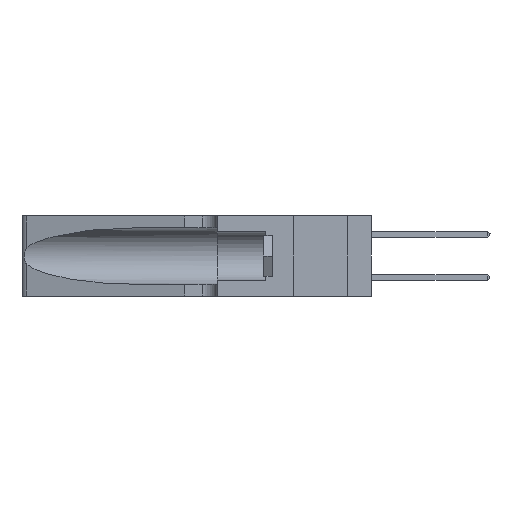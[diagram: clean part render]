
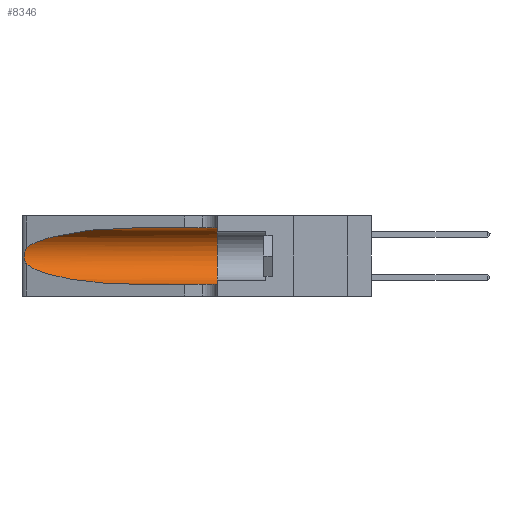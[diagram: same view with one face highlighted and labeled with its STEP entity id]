
A CAD part, left-side view. The second image highlights one B-rep face of the part: STEP entity #8346.
In plain terms, the highlighted cylindrical face has radius 3.308 mm (diameter 6.617 mm), a partial arc.
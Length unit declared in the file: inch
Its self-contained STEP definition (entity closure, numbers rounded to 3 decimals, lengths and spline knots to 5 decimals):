
#1236 = CARTESIAN_POINT ( 'NONE',  ( 0.25639, 1.23184, 0.21858 ) ) ;
#1333 =( BOUNDED_CURVE ( )  B_SPLINE_CURVE ( 3, ( #10373, #8876, #10526, #2086 ),
 .UNSPECIFIED., .F., .T. ) 
 B_SPLINE_CURVE_WITH_KNOTS ( ( 4, 4 ),
 ( 3.44316, 4.71239 ),
 .UNSPECIFIED. ) 
 CURVE ( )  GEOMETRIC_REPRESENTATION_ITEM ( )  RATIONAL_B_SPLINE_CURVE ( ( 1., 0.87, 0.87, 1. ) ) 
 REPRESENTATION_ITEM ( '' )  );
#1506 = CARTESIAN_POINT ( 'NONE',  ( 0.1305, 0.35, 0.185 ) ) ;
#1626 = AXIS2_PLACEMENT_3D ( 'NONE', #2397, #3921, #17804 ) ;
#1773 = CARTESIAN_POINT ( 'NONE',  ( 0.1305, 0.72297, 0.31525 ) ) ;
#2086 = CARTESIAN_POINT ( 'NONE',  ( 0.1305, 0.72297, 0.05475 ) ) ;
#2121 = ORIENTED_EDGE ( 'NONE', *, *, #9922, .T. ) ;
#2397 = CARTESIAN_POINT ( 'NONE',  ( 0.1305, 1.61858, 0.185 ) ) ;
#2415 = VERTEX_POINT ( 'NONE', #15069 ) ;
#2681 = CARTESIAN_POINT ( 'NONE',  ( 0.1305, 0.72297, 0.31525 ) ) ;
#2907 = CARTESIAN_POINT ( 'NONE',  ( 0.1305, 0.35, 0.31525 ) ) ;
#3198 = CARTESIAN_POINT ( 'NONE',  ( 0.26075, 1.23896, 0.19203 ) ) ;
#3245 = DIRECTION ( 'NONE',  ( 0., 0., 1. ) ) ;
#3446 = CARTESIAN_POINT ( 'NONE',  ( 0.2373, 1.15595, 0.28018 ) ) ;
#3921 = DIRECTION ( 'NONE',  ( 0., -1., 0. ) ) ;
#3967 =( BOUNDED_CURVE ( )  B_SPLINE_CURVE ( 3, ( #1773, #13787, #3446, #15420 ),
 .UNSPECIFIED., .F., .T. ) 
 B_SPLINE_CURVE_WITH_KNOTS ( ( 4, 4 ),
 ( 1.5708, 2.84003 ),
 .UNSPECIFIED. ) 
 CURVE ( )  GEOMETRIC_REPRESENTATION_ITEM ( )  RATIONAL_B_SPLINE_CURVE ( ( 1., 0.87, 0.87, 1. ) ) 
 REPRESENTATION_ITEM ( '' )  );
#4155 = EDGE_CURVE ( 'NONE', #12718, #6421, #21612, .T. ) ;
#4367 = ORIENTED_EDGE ( 'NONE', *, *, #4155, .T. ) ;
#4467 = CARTESIAN_POINT ( 'NONE',  ( 0.25487, 1.22718, 0.22369 ) ) ;
#4533 = CARTESIAN_POINT ( 'NONE',  ( 0.25555, 1.22994, 0.2215 ) ) ;
#4665 = VECTOR ( 'NONE', #13115, 39.37008 ) ;
#4834 = AXIS2_PLACEMENT_3D ( 'NONE', #1506, #13512, #3245 ) ;
#6277 = CARTESIAN_POINT ( 'NONE',  ( 0.1305, 1.61858, 0.05475 ) ) ;
#6398 = CARTESIAN_POINT ( 'NONE',  ( 0.26018, 1.23835, 0.19895 ) ) ;
#6421 = VERTEX_POINT ( 'NONE', #19891 ) ;
#6625 = CARTESIAN_POINT ( 'NONE',  ( 0.26017, 1.23833, 0.17102 ) ) ;
#7661 = ORIENTED_EDGE ( 'NONE', *, *, #12439, .F. ) ;
#8099 = LINE ( 'NONE', #6277, #4665 ) ;
#8321 = CARTESIAN_POINT ( 'NONE',  ( 0.25856, 1.23593, 0.16098 ) ) ;
#8346 = ADVANCED_FACE ( 'NONE', ( #17374 ), #18987, .F. ) ;
#8475 = EDGE_LOOP ( 'NONE', ( #17285, #4367, #2121, #21771, #7661, #13312 ) ) ;
#8876 = CARTESIAN_POINT ( 'NONE',  ( 0.2373, 1.15595, 0.08982 ) ) ;
#9891 = CIRCLE ( 'NONE', #4834, 0.13025 ) ;
#9922 = EDGE_CURVE ( 'NONE', #6421, #16425, #1333, .T. ) ;
#10373 = CARTESIAN_POINT ( 'NONE',  ( 0.25487, 1.22718, 0.14631 ) ) ;
#10526 = CARTESIAN_POINT ( 'NONE',  ( 0.18966, 0.96281, 0.05475 ) ) ;
#10617 = EDGE_CURVE ( 'NONE', #16425, #2415, #8099, .T. ) ;
#11741 = VECTOR ( 'NONE', #16074, 39.37008 ) ;
#11746 = LINE ( 'NONE', #17626, #11741 ) ;
#12439 = EDGE_CURVE ( 'NONE', #13881, #2415, #9891, .T. ) ;
#12718 = VERTEX_POINT ( 'NONE', #21717 ) ;
#13115 = DIRECTION ( 'NONE',  ( 0., -1., 0. ) ) ;
#13312 = ORIENTED_EDGE ( 'NONE', *, *, #20594, .F. ) ;
#13512 = DIRECTION ( 'NONE',  ( 0., 1., 0. ) ) ;
#13787 = CARTESIAN_POINT ( 'NONE',  ( 0.18966, 0.96281, 0.31525 ) ) ;
#13881 = VERTEX_POINT ( 'NONE', #2907 ) ;
#14976 = CARTESIAN_POINT ( 'NONE',  ( 0.25787, 1.23484, 0.2124 ) ) ;
#15069 = CARTESIAN_POINT ( 'NONE',  ( 0.1305, 0.35, 0.05475 ) ) ;
#15420 = CARTESIAN_POINT ( 'NONE',  ( 0.25487, 1.22718, 0.22369 ) ) ;
#16074 = DIRECTION ( 'NONE',  ( 0., -1., 0. ) ) ;
#16425 = VERTEX_POINT ( 'NONE', #20793 ) ;
#16427 = EDGE_CURVE ( 'NONE', #21908, #12718, #3967, .T. ) ;
#16692 = CARTESIAN_POINT ( 'NONE',  ( 0.25854, 1.2359, 0.20912 ) ) ;
#17285 = ORIENTED_EDGE ( 'NONE', *, *, #16427, .T. ) ;
#17374 = FACE_OUTER_BOUND ( 'NONE', #8475, .T. ) ;
#17626 = CARTESIAN_POINT ( 'NONE',  ( 0.1305, 1.61858, 0.31525 ) ) ;
#17804 = DIRECTION ( 'NONE',  ( 0., 0., -1. ) ) ;
#18987 = CYLINDRICAL_SURFACE ( 'NONE', #1626, 0.13025 ) ;
#19483 = CARTESIAN_POINT ( 'NONE',  ( 0.25487, 1.22718, 0.14631 ) ) ;
#19891 = CARTESIAN_POINT ( 'NONE',  ( 0.25487, 1.22718, 0.14631 ) ) ;
#20402 = CARTESIAN_POINT ( 'NONE',  ( 0.25639, 1.23186, 0.15144 ) ) ;
#20594 = EDGE_CURVE ( 'NONE', #21908, #13881, #11746, .T. ) ;
#20793 = CARTESIAN_POINT ( 'NONE',  ( 0.1305, 0.72297, 0.05475 ) ) ;
#21612 = B_SPLINE_CURVE_WITH_KNOTS ( 'NONE', 3,
 ( #4467, #4533, #1236, #14976, #16692, #6398, #3198, #22231, #6625, #8321, #21933, #20402, #22148, #19483 ),
 .UNSPECIFIED., .F., .F.,
 ( 4, 2, 2, 2, 2, 2, 4 ),
 ( 0., 0.00027, 0.00053, 0.00107, 0.0016, 0.00187, 0.00214 ),
 .UNSPECIFIED. ) ;
#21717 = CARTESIAN_POINT ( 'NONE',  ( 0.25487, 1.22718, 0.22369 ) ) ;
#21771 = ORIENTED_EDGE ( 'NONE', *, *, #10617, .T. ) ;
#21908 = VERTEX_POINT ( 'NONE', #2681 ) ;
#21933 = CARTESIAN_POINT ( 'NONE',  ( 0.25789, 1.23486, 0.15765 ) ) ;
#22148 = CARTESIAN_POINT ( 'NONE',  ( 0.25555, 1.22993, 0.14849 ) ) ;
#22231 = CARTESIAN_POINT ( 'NONE',  ( 0.26075, 1.23896, 0.178 ) ) ;
